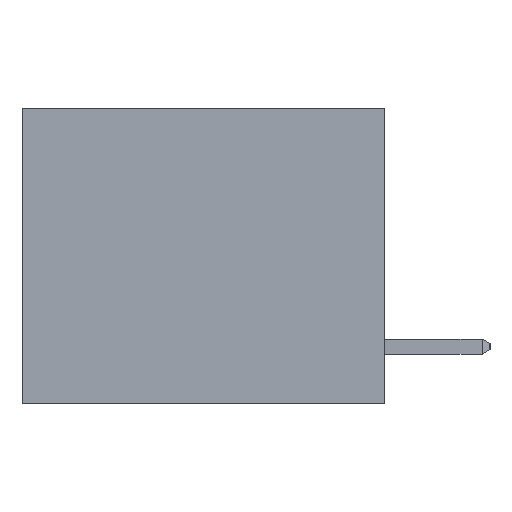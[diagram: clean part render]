
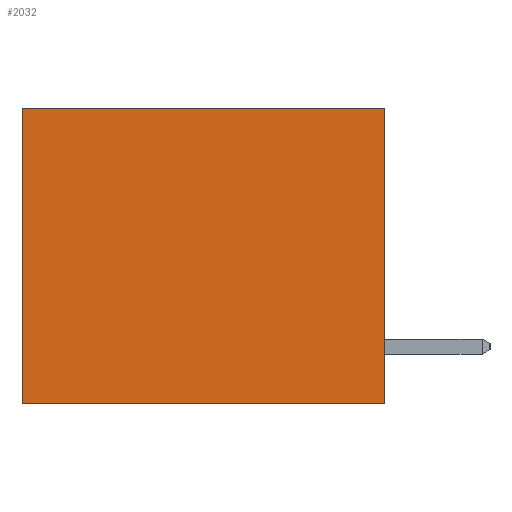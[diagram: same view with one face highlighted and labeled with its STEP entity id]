
A CAD part, left-side view. The second image highlights one B-rep face of the part: STEP entity #2032.
In plain terms, the highlighted planar face has unit normal (-1, 0, 0).
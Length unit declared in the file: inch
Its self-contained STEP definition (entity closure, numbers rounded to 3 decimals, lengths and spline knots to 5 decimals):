
#113 = EDGE_CURVE ( 'NONE', #9695, #8868, #2748, .T. ) ;
#280 = VECTOR ( 'NONE', #2850, 39.37008 ) ;
#835 = DIRECTION ( 'NONE',  ( 0., 1., 0. ) ) ;
#886 = EDGE_CURVE ( 'NONE', #8868, #6464, #4495, .T. ) ;
#953 = CARTESIAN_POINT ( 'NONE',  ( 0.3165, 0., -0.49 ) ) ;
#1478 = EDGE_CURVE ( 'NONE', #9695, #5372, #10902, .T. ) ;
#1743 = DIRECTION ( 'NONE',  ( 1., 0., 0. ) ) ;
#2032 = ADVANCED_FACE ( 'NONE', ( #12095 ), #10740, .F. ) ;
#2333 = VECTOR ( 'NONE', #9229, 39.37008 ) ;
#2416 = VECTOR ( 'NONE', #3061, 39.37008 ) ;
#2748 = LINE ( 'NONE', #953, #2416 ) ;
#2850 = DIRECTION ( 'NONE',  ( 0., 1., 0. ) ) ;
#3061 = DIRECTION ( 'NONE',  ( 0., 0., -1. ) ) ;
#3256 = CARTESIAN_POINT ( 'NONE',  ( 0.3165, 0.6, 0. ) ) ;
#3280 = AXIS2_PLACEMENT_3D ( 'NONE', #11638, #1743, #3760 ) ;
#3760 = DIRECTION ( 'NONE',  ( 0., 0., -1. ) ) ;
#3917 = CARTESIAN_POINT ( 'NONE',  ( 0.3165, 0., -0.49 ) ) ;
#4295 = CARTESIAN_POINT ( 'NONE',  ( 0.3165, 0., -0.49 ) ) ;
#4364 = ORIENTED_EDGE ( 'NONE', *, *, #886, .F. ) ;
#4495 = LINE ( 'NONE', #3917, #8402 ) ;
#4999 = LINE ( 'NONE', #6303, #2333 ) ;
#5372 = VERTEX_POINT ( 'NONE', #3256 ) ;
#5649 = CARTESIAN_POINT ( 'NONE',  ( 0.3165, 0., 0. ) ) ;
#5694 = CARTESIAN_POINT ( 'NONE',  ( 0.3165, 0.6, -0.49 ) ) ;
#5921 = EDGE_CURVE ( 'NONE', #5372, #6464, #4999, .T. ) ;
#6303 = CARTESIAN_POINT ( 'NONE',  ( 0.3165, 0.6, -0.49 ) ) ;
#6464 = VERTEX_POINT ( 'NONE', #5694 ) ;
#6818 = ORIENTED_EDGE ( 'NONE', *, *, #1478, .T. ) ;
#8402 = VECTOR ( 'NONE', #835, 39.37008 ) ;
#8868 = VERTEX_POINT ( 'NONE', #4295 ) ;
#9229 = DIRECTION ( 'NONE',  ( 0., 0., -1. ) ) ;
#9695 = VERTEX_POINT ( 'NONE', #10293 ) ;
#10293 = CARTESIAN_POINT ( 'NONE',  ( 0.3165, 0., 0. ) ) ;
#10740 = PLANE ( 'NONE',  #3280 ) ;
#10902 = LINE ( 'NONE', #5649, #280 ) ;
#11587 = EDGE_LOOP ( 'NONE', ( #11833, #4364, #12548, #6818 ) ) ;
#11638 = CARTESIAN_POINT ( 'NONE',  ( 0.3165, 0., -0.49 ) ) ;
#11833 = ORIENTED_EDGE ( 'NONE', *, *, #5921, .T. ) ;
#12095 = FACE_OUTER_BOUND ( 'NONE', #11587, .T. ) ;
#12548 = ORIENTED_EDGE ( 'NONE', *, *, #113, .F. ) ;
